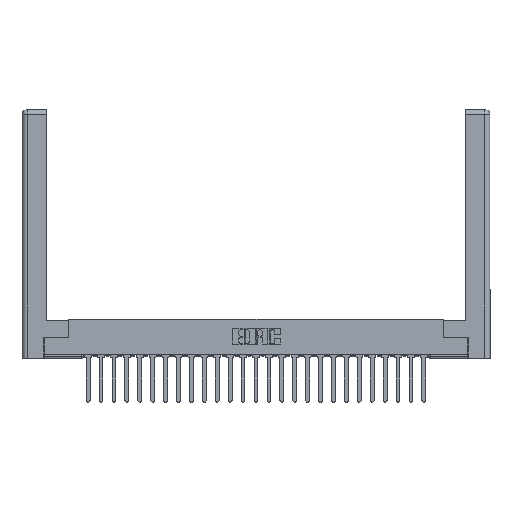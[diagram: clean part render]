
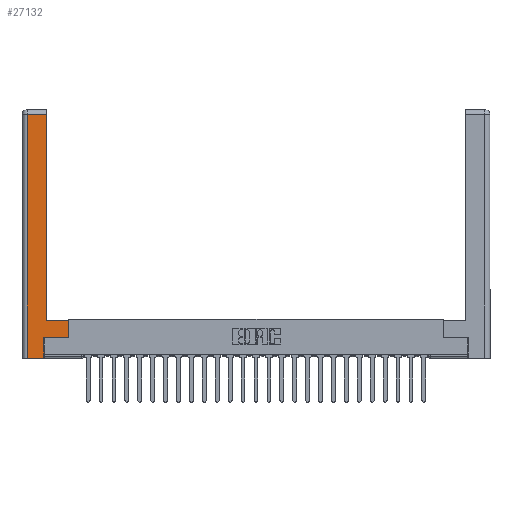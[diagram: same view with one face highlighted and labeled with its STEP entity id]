
A CAD part, top view. The second image highlights one B-rep face of the part: STEP entity #27132.
In plain terms, the highlighted planar face has unit normal (0, 0, 1).
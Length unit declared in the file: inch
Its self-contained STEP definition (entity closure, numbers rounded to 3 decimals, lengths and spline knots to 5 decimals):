
#17 = CARTESIAN_POINT ( 'NONE',  ( 0.295, 0.45, 0. ) ) ;
#1118 = CARTESIAN_POINT ( 'NONE',  ( 0.0615, 0., 0. ) ) ;
#1154 = VERTEX_POINT ( 'NONE', #15934 ) ;
#1181 = EDGE_CURVE ( 'NONE', #11025, #19183, #25078, .T. ) ;
#1830 = EDGE_CURVE ( 'NONE', #25073, #16598, #14655, .T. ) ;
#3088 = ORIENTED_EDGE ( 'NONE', *, *, #1830, .T. ) ;
#3427 = DIRECTION ( 'NONE',  ( -1., 0., 0. ) ) ;
#3478 = VECTOR ( 'NONE', #5299, 39.37008 ) ;
#3570 = VECTOR ( 'NONE', #3854, 39.37008 ) ;
#3854 = DIRECTION ( 'NONE',  ( 0., 1., 0. ) ) ;
#3935 = CARTESIAN_POINT ( 'NONE',  ( 0.565, 0.45, 0. ) ) ;
#4393 = CARTESIAN_POINT ( 'NONE',  ( 0., 0., 0. ) ) ;
#4468 = EDGE_CURVE ( 'NONE', #19183, #1154, #7180, .T. ) ;
#4966 = VECTOR ( 'NONE', #3427, 39.37008 ) ;
#5299 = DIRECTION ( 'NONE',  ( 0., -1., 0. ) ) ;
#6249 = DIRECTION ( 'NONE',  ( 1., 0., 0. ) ) ;
#6515 = PLANE ( 'NONE',  #14022 ) ;
#6530 = CARTESIAN_POINT ( 'NONE',  ( 0.565, 0.45, 0. ) ) ;
#7132 = EDGE_CURVE ( 'NONE', #24820, #11025, #11134, .T. ) ;
#7180 = LINE ( 'NONE', #19227, #27237 ) ;
#7783 = CARTESIAN_POINT ( 'NONE',  ( 0.0615, 2.94, 0. ) ) ;
#8089 = VECTOR ( 'NONE', #6249, 39.37008 ) ;
#8358 = ORIENTED_EDGE ( 'NONE', *, *, #7132, .T. ) ;
#8468 = CARTESIAN_POINT ( 'NONE',  ( 0.0615, 0., 0. ) ) ;
#10665 = DIRECTION ( 'NONE',  ( 0., 1., 0. ) ) ;
#10790 = EDGE_LOOP ( 'NONE', ( #3088, #19168, #8358, #20008, #13055, #17236, #19087, #15532 ) ) ;
#10813 = DIRECTION ( 'NONE',  ( 0., 0., -1. ) ) ;
#10988 = VECTOR ( 'NONE', #17859, 39.37008 ) ;
#11025 = VERTEX_POINT ( 'NONE', #8468 ) ;
#11134 = LINE ( 'NONE', #1118, #3478 ) ;
#11455 = CARTESIAN_POINT ( 'NONE',  ( 0.295, 0.45, 0. ) ) ;
#11576 = FACE_OUTER_BOUND ( 'NONE', #10790, .T. ) ;
#12957 = DIRECTION ( 'NONE',  ( -1., 0., 0. ) ) ;
#13055 = ORIENTED_EDGE ( 'NONE', *, *, #4468, .T. ) ;
#13696 = CARTESIAN_POINT ( 'NONE',  ( 0.0615, 2.94, 0. ) ) ;
#14022 = AXIS2_PLACEMENT_3D ( 'NONE', #4393, #10813, #12957 ) ;
#14655 = LINE ( 'NONE', #20390, #10988 ) ;
#15532 = ORIENTED_EDGE ( 'NONE', *, *, #22925, .T. ) ;
#15577 = LINE ( 'NONE', #11455, #20278 ) ;
#15844 = DIRECTION ( 'NONE',  ( 1., 0., 0. ) ) ;
#15934 = CARTESIAN_POINT ( 'NONE',  ( 0.265, 0.245, 0. ) ) ;
#16385 = VERTEX_POINT ( 'NONE', #24155 ) ;
#16598 = VERTEX_POINT ( 'NONE', #20313 ) ;
#17014 = EDGE_CURVE ( 'NONE', #1154, #16385, #26472, .T. ) ;
#17015 = VECTOR ( 'NONE', #15844, 39.37008 ) ;
#17236 = ORIENTED_EDGE ( 'NONE', *, *, #17014, .T. ) ;
#17859 = DIRECTION ( 'NONE',  ( 0., 1., 0. ) ) ;
#17932 = LINE ( 'NONE', #7783, #4966 ) ;
#19005 = CARTESIAN_POINT ( 'NONE',  ( 0.565, 0.245, 0. ) ) ;
#19087 = ORIENTED_EDGE ( 'NONE', *, *, #26932, .T. ) ;
#19168 = ORIENTED_EDGE ( 'NONE', *, *, #22476, .T. ) ;
#19183 = VERTEX_POINT ( 'NONE', #25196 ) ;
#19227 = CARTESIAN_POINT ( 'NONE',  ( 0.265, 0.245, 0. ) ) ;
#20008 = ORIENTED_EDGE ( 'NONE', *, *, #1181, .T. ) ;
#20278 = VECTOR ( 'NONE', #21992, 39.37008 ) ;
#20313 = CARTESIAN_POINT ( 'NONE',  ( 0.295, 2.94, 0. ) ) ;
#20390 = CARTESIAN_POINT ( 'NONE',  ( 0.295, 3., 0. ) ) ;
#21992 = DIRECTION ( 'NONE',  ( -1., 0., 0. ) ) ;
#22476 = EDGE_CURVE ( 'NONE', #16598, #24820, #17932, .T. ) ;
#22925 = EDGE_CURVE ( 'NONE', #24524, #25073, #15577, .T. ) ;
#24155 = CARTESIAN_POINT ( 'NONE',  ( 0.565, 0.245, 0. ) ) ;
#24460 = CARTESIAN_POINT ( 'NONE',  ( 0.265, 0., 0. ) ) ;
#24524 = VERTEX_POINT ( 'NONE', #6530 ) ;
#24820 = VERTEX_POINT ( 'NONE', #13696 ) ;
#25073 = VERTEX_POINT ( 'NONE', #17 ) ;
#25078 = LINE ( 'NONE', #24460, #17015 ) ;
#25196 = CARTESIAN_POINT ( 'NONE',  ( 0.265, 0., 0. ) ) ;
#26472 = LINE ( 'NONE', #19005, #8089 ) ;
#26932 = EDGE_CURVE ( 'NONE', #16385, #24524, #27251, .T. ) ;
#27132 = ADVANCED_FACE ( 'NONE', ( #11576 ), #6515, .F. ) ;
#27237 = VECTOR ( 'NONE', #10665, 39.37008 ) ;
#27251 = LINE ( 'NONE', #3935, #3570 ) ;
